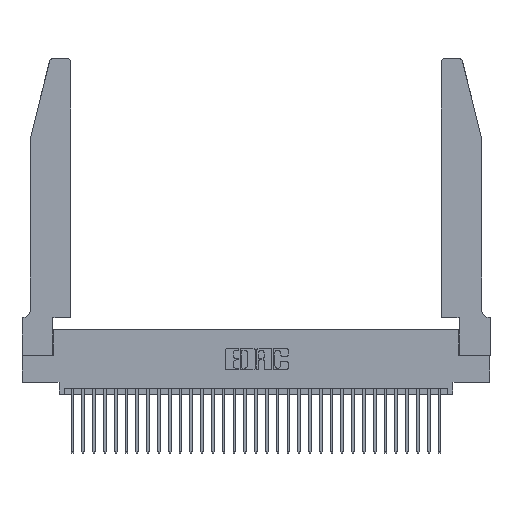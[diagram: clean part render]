
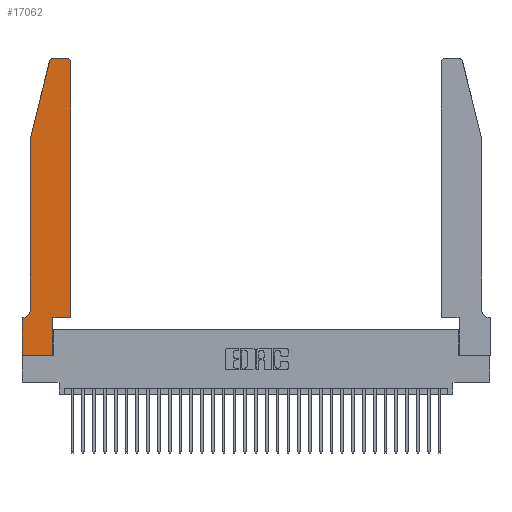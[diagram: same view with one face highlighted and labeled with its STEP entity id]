
A CAD part, top view. The second image highlights one B-rep face of the part: STEP entity #17062.
In plain terms, the highlighted planar face has unit normal (0, 0, 1).
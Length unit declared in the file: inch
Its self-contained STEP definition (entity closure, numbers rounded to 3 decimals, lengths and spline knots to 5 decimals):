
#304 = ORIENTED_EDGE ( 'NONE', *, *, #26582, .T. ) ;
#1293 = CIRCLE ( 'NONE', #20338, 0.07 ) ;
#1430 = EDGE_CURVE ( 'NONE', #16726, #10782, #6116, .T. ) ;
#1611 = VERTEX_POINT ( 'NONE', #14636 ) ;
#1763 = EDGE_CURVE ( 'NONE', #12220, #2858, #17372, .T. ) ;
#1876 = DIRECTION ( 'NONE',  ( 0., 0., 1. ) ) ;
#1992 = CARTESIAN_POINT ( 'NONE',  ( 0.4505, 0.35, 0.37 ) ) ;
#2814 = VERTEX_POINT ( 'NONE', #19849 ) ;
#2858 = VERTEX_POINT ( 'NONE', #28267 ) ;
#3368 = VECTOR ( 'NONE', #20460, 39.37008 ) ;
#4807 = CARTESIAN_POINT ( 'NONE',  ( 0.0755, 2., 0.37 ) ) ;
#5048 = CARTESIAN_POINT ( 'NONE',  ( 0.0755, 2., 0.37 ) ) ;
#5090 = ORIENTED_EDGE ( 'NONE', *, *, #5592, .T. ) ;
#5582 = LINE ( 'NONE', #13646, #32547 ) ;
#5592 = EDGE_CURVE ( 'NONE', #11892, #2814, #7093, .T. ) ;
#5981 = CARTESIAN_POINT ( 'NONE',  ( 0.0755, 2., 0.37 ) ) ;
#6079 = CARTESIAN_POINT ( 'NONE',  ( 0.2865, 0.35, 0.37 ) ) ;
#6116 = LINE ( 'NONE', #6079, #7727 ) ;
#6194 = VECTOR ( 'NONE', #21668, 39.37008 ) ;
#6209 = DIRECTION ( 'NONE',  ( 0., 0., 1. ) ) ;
#6395 = VERTEX_POINT ( 'NONE', #18246 ) ;
#6484 = DIRECTION ( 'NONE',  ( 0., 0., 1. ) ) ;
#7093 = LINE ( 'NONE', #18272, #32832 ) ;
#7727 = VECTOR ( 'NONE', #31843, 39.37008 ) ;
#7782 = DIRECTION ( 'NONE',  ( -1., 0., 0. ) ) ;
#7796 = LINE ( 'NONE', #5048, #3368 ) ;
#8271 = VERTEX_POINT ( 'NONE', #27059 ) ;
#9748 = DIRECTION ( 'NONE',  ( -1., 0., 0. ) ) ;
#10782 = VERTEX_POINT ( 'NONE', #28652 ) ;
#11301 = VECTOR ( 'NONE', #16974, 39.37008 ) ;
#11674 = ORIENTED_EDGE ( 'NONE', *, *, #12055, .T. ) ;
#11857 = PLANE ( 'NONE',  #21227 ) ;
#11892 = VERTEX_POINT ( 'NONE', #19010 ) ;
#12055 = EDGE_CURVE ( 'NONE', #16220, #32868, #27904, .T. ) ;
#12220 = VERTEX_POINT ( 'NONE', #5981 ) ;
#12251 = CARTESIAN_POINT ( 'NONE',  ( 0.0055, 0.42, 0.37 ) ) ;
#12995 = CARTESIAN_POINT ( 'NONE',  ( 0.4505, 2.72, 0.37 ) ) ;
#13012 = DIRECTION ( 'NONE',  ( 1., 0., 0. ) ) ;
#13128 = CARTESIAN_POINT ( 'NONE',  ( 0.4205, 2.72, 0.37 ) ) ;
#13575 = ORIENTED_EDGE ( 'NONE', *, *, #26238, .T. ) ;
#13646 = CARTESIAN_POINT ( 'NONE',  ( 0.0755, 0.35, 0.37 ) ) ;
#13808 = VECTOR ( 'NONE', #19781, 39.37008 ) ;
#14212 = EDGE_CURVE ( 'NONE', #2814, #16726, #22989, .T. ) ;
#14636 = CARTESIAN_POINT ( 'NONE',  ( 0.4505, 0.35, 0.37 ) ) ;
#15752 = ORIENTED_EDGE ( 'NONE', *, *, #17417, .T. ) ;
#15893 = AXIS2_PLACEMENT_3D ( 'NONE', #13128, #6484, #13012 ) ;
#15970 = EDGE_CURVE ( 'NONE', #2858, #8271, #1293, .T. ) ;
#16211 = CARTESIAN_POINT ( 'NONE',  ( 0.2865, 0., 0.37 ) ) ;
#16220 = VERTEX_POINT ( 'NONE', #29213 ) ;
#16565 = VECTOR ( 'NONE', #25416, 39.37008 ) ;
#16584 = CARTESIAN_POINT ( 'NONE',  ( 0.284, 2.72, 0.37 ) ) ;
#16726 = VERTEX_POINT ( 'NONE', #16211 ) ;
#16974 = DIRECTION ( 'NONE',  ( 1., 0., 0. ) ) ;
#17062 = ADVANCED_FACE ( 'NONE', ( #22887 ), #11857, .T. ) ;
#17312 = CARTESIAN_POINT ( 'NONE',  ( 0., 0.35, 0.37 ) ) ;
#17372 = LINE ( 'NONE', #4807, #16565 ) ;
#17410 = ORIENTED_EDGE ( 'NONE', *, *, #20184, .T. ) ;
#17417 = EDGE_CURVE ( 'NONE', #8271, #11892, #5582, .T. ) ;
#18017 = DIRECTION ( 'NONE',  ( 0., 0., -1. ) ) ;
#18246 = CARTESIAN_POINT ( 'NONE',  ( 0.25487, 2.72718, 0.37 ) ) ;
#18272 = CARTESIAN_POINT ( 'NONE',  ( 0., 0., 0.37 ) ) ;
#18900 = VECTOR ( 'NONE', #19895, 39.37008 ) ;
#19010 = CARTESIAN_POINT ( 'NONE',  ( 0., 0.35, 0.37 ) ) ;
#19080 = CARTESIAN_POINT ( 'NONE',  ( 0.4505, 0.35, 0.37 ) ) ;
#19781 = DIRECTION ( 'NONE',  ( 0., 1., 0. ) ) ;
#19849 = CARTESIAN_POINT ( 'NONE',  ( 0., 0., 0.37 ) ) ;
#19895 = DIRECTION ( 'NONE',  ( 1., 0., 0. ) ) ;
#20184 = EDGE_CURVE ( 'NONE', #32868, #6395, #29986, .T. ) ;
#20338 = AXIS2_PLACEMENT_3D ( 'NONE', #12251, #18017, #7782 ) ;
#20460 = DIRECTION ( 'NONE',  ( -0.239, -0.971, 0. ) ) ;
#20885 = DIRECTION ( 'NONE',  ( 0., -1., 0. ) ) ;
#21097 = CIRCLE ( 'NONE', #15893, 0.03 ) ;
#21227 = AXIS2_PLACEMENT_3D ( 'NONE', #17312, #1876, #29887 ) ;
#21668 = DIRECTION ( 'NONE',  ( -1., 0., 0. ) ) ;
#21737 = ORIENTED_EDGE ( 'NONE', *, *, #32649, .T. ) ;
#21976 = EDGE_LOOP ( 'NONE', ( #11674, #17410, #13575, #30656, #25361, #15752, #5090, #24396, #31287, #24079, #304, #21737 ) ) ;
#21986 = CARTESIAN_POINT ( 'NONE',  ( 0., 0., 0.37 ) ) ;
#22887 = FACE_OUTER_BOUND ( 'NONE', #21976, .T. ) ;
#22976 = EDGE_CURVE ( 'NONE', #10782, #1611, #25747, .T. ) ;
#22989 = LINE ( 'NONE', #21986, #11301 ) ;
#24079 = ORIENTED_EDGE ( 'NONE', *, *, #22976, .T. ) ;
#24396 = ORIENTED_EDGE ( 'NONE', *, *, #14212, .T. ) ;
#25361 = ORIENTED_EDGE ( 'NONE', *, *, #15970, .T. ) ;
#25416 = DIRECTION ( 'NONE',  ( 0., -1., 0. ) ) ;
#25747 = LINE ( 'NONE', #1992, #18900 ) ;
#26238 = EDGE_CURVE ( 'NONE', #6395, #12220, #7796, .T. ) ;
#26405 = VERTEX_POINT ( 'NONE', #12995 ) ;
#26582 = EDGE_CURVE ( 'NONE', #1611, #26405, #29090, .T. ) ;
#27059 = CARTESIAN_POINT ( 'NONE',  ( 0.0055, 0.35, 0.37 ) ) ;
#27163 = CARTESIAN_POINT ( 'NONE',  ( 0.2605, 2.75, 0.37 ) ) ;
#27904 = LINE ( 'NONE', #27163, #6194 ) ;
#28267 = CARTESIAN_POINT ( 'NONE',  ( 0.0755, 0.42, 0.37 ) ) ;
#28652 = CARTESIAN_POINT ( 'NONE',  ( 0.2865, 0.35, 0.37 ) ) ;
#28764 = CARTESIAN_POINT ( 'NONE',  ( 0.284, 2.75, 0.37 ) ) ;
#29090 = LINE ( 'NONE', #19080, #13808 ) ;
#29149 = DIRECTION ( 'NONE',  ( 1., 0., 0. ) ) ;
#29213 = CARTESIAN_POINT ( 'NONE',  ( 0.4205, 2.75, 0.37 ) ) ;
#29887 = DIRECTION ( 'NONE',  ( 1., 0., 0. ) ) ;
#29986 = CIRCLE ( 'NONE', #30526, 0.03 ) ;
#30526 = AXIS2_PLACEMENT_3D ( 'NONE', #16584, #6209, #29149 ) ;
#30656 = ORIENTED_EDGE ( 'NONE', *, *, #1763, .T. ) ;
#31287 = ORIENTED_EDGE ( 'NONE', *, *, #1430, .T. ) ;
#31843 = DIRECTION ( 'NONE',  ( 0., 1., 0. ) ) ;
#32547 = VECTOR ( 'NONE', #9748, 39.37008 ) ;
#32649 = EDGE_CURVE ( 'NONE', #26405, #16220, #21097, .T. ) ;
#32832 = VECTOR ( 'NONE', #20885, 39.37008 ) ;
#32868 = VERTEX_POINT ( 'NONE', #28764 ) ;
